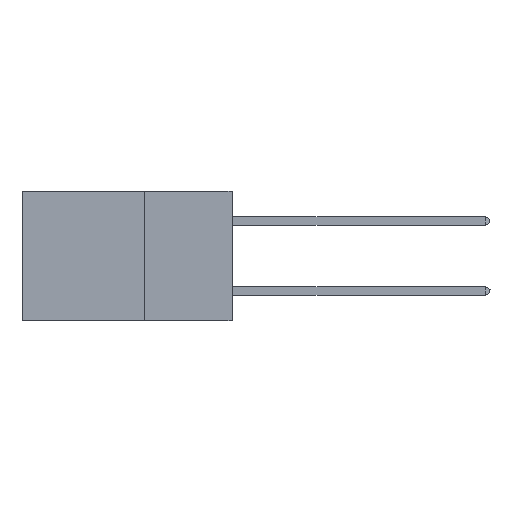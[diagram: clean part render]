
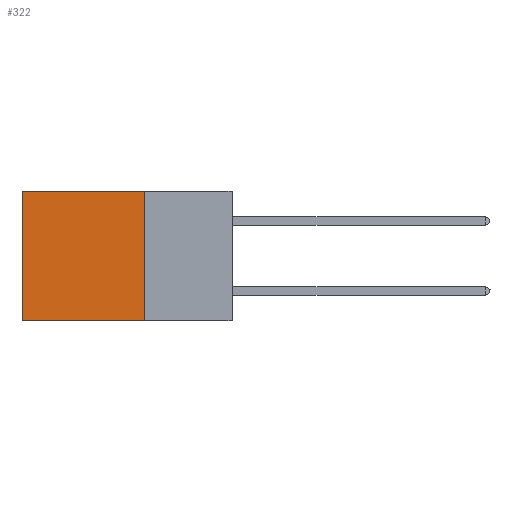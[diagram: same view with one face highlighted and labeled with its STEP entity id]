
A CAD part, left-side view. The second image highlights one B-rep face of the part: STEP entity #322.
In plain terms, the highlighted planar face has unit normal (-1, 0, 0).
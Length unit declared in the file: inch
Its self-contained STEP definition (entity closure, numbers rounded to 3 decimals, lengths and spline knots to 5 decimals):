
#322 = ADVANCED_FACE ( 'NONE', ( #25251 ), #1339, .F. ) ;
#1339 = PLANE ( 'NONE',  #1915 ) ;
#1854 = CARTESIAN_POINT ( 'NONE',  ( 0.2875, 0.25, 0. ) ) ;
#1915 = AXIS2_PLACEMENT_3D ( 'NONE', #10114, #23669, #5551 ) ;
#2150 = VERTEX_POINT ( 'NONE', #4843 ) ;
#3096 = EDGE_CURVE ( 'NONE', #15964, #12830, #26148, .T. ) ;
#4843 = CARTESIAN_POINT ( 'NONE',  ( 0.2875, 0.25, 0. ) ) ;
#5060 = VECTOR ( 'NONE', #28086, 39.37008 ) ;
#5551 = DIRECTION ( 'NONE',  ( 0., 0., -1. ) ) ;
#7231 = DIRECTION ( 'NONE',  ( 0., 1., 0. ) ) ;
#9750 = VECTOR ( 'NONE', #18109, 39.37008 ) ;
#10114 = CARTESIAN_POINT ( 'NONE',  ( 0.2875, 0.25, 0. ) ) ;
#11893 = ORIENTED_EDGE ( 'NONE', *, *, #3096, .F. ) ;
#11979 = VERTEX_POINT ( 'NONE', #27419 ) ;
#12652 = EDGE_CURVE ( 'NONE', #11979, #12830, #17366, .T. ) ;
#12779 = ORIENTED_EDGE ( 'NONE', *, *, #27692, .T. ) ;
#12830 = VERTEX_POINT ( 'NONE', #15176 ) ;
#13563 = EDGE_LOOP ( 'NONE', ( #16886, #11893, #26854, #12779 ) ) ;
#14810 = CARTESIAN_POINT ( 'NONE',  ( 0.2875, 0.25, -0.37 ) ) ;
#15176 = CARTESIAN_POINT ( 'NONE',  ( 0.2875, 0.6, -0.37 ) ) ;
#15964 = VERTEX_POINT ( 'NONE', #14810 ) ;
#16886 = ORIENTED_EDGE ( 'NONE', *, *, #12652, .T. ) ;
#17241 = CARTESIAN_POINT ( 'NONE',  ( 0.2875, 0.25, -0.37 ) ) ;
#17366 = LINE ( 'NONE', #25949, #5060 ) ;
#18109 = DIRECTION ( 'NONE',  ( 0., 0., -1. ) ) ;
#18683 = CARTESIAN_POINT ( 'NONE',  ( 0.2875, 0.25, 0. ) ) ;
#21309 = VECTOR ( 'NONE', #7231, 39.37008 ) ;
#23669 = DIRECTION ( 'NONE',  ( 1., 0., 0. ) ) ;
#24345 = EDGE_CURVE ( 'NONE', #2150, #15964, #27056, .T. ) ;
#25251 = FACE_OUTER_BOUND ( 'NONE', #13563, .T. ) ;
#25426 = VECTOR ( 'NONE', #28370, 39.37008 ) ;
#25949 = CARTESIAN_POINT ( 'NONE',  ( 0.2875, 0.6, 0. ) ) ;
#26148 = LINE ( 'NONE', #17241, #25426 ) ;
#26510 = LINE ( 'NONE', #18683, #21309 ) ;
#26854 = ORIENTED_EDGE ( 'NONE', *, *, #24345, .F. ) ;
#27056 = LINE ( 'NONE', #1854, #9750 ) ;
#27419 = CARTESIAN_POINT ( 'NONE',  ( 0.2875, 0.6, 0. ) ) ;
#27692 = EDGE_CURVE ( 'NONE', #2150, #11979, #26510, .T. ) ;
#28086 = DIRECTION ( 'NONE',  ( 0., 0., -1. ) ) ;
#28370 = DIRECTION ( 'NONE',  ( 0., 1., 0. ) ) ;
